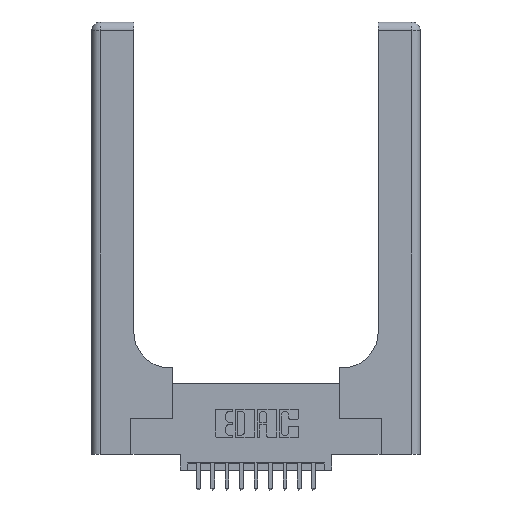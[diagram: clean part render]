
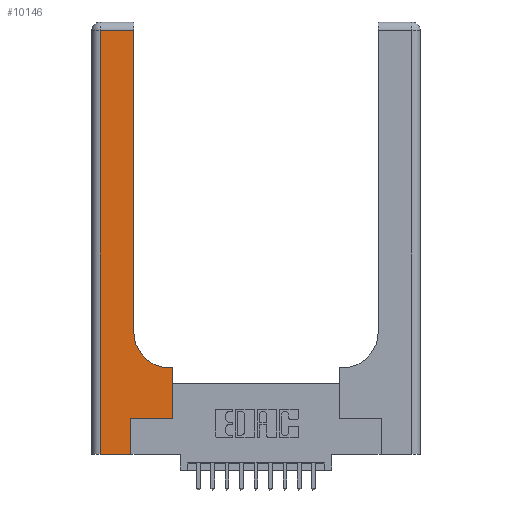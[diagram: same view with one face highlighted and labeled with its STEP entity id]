
A CAD part, top view. The second image highlights one B-rep face of the part: STEP entity #10146.
In plain terms, the highlighted planar face has unit normal (0, 0, 1).
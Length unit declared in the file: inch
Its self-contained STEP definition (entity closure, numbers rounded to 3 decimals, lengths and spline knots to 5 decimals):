
#248 = CARTESIAN_POINT ( 'NONE',  ( 0., 3., 0.37 ) ) ;
#299 = CARTESIAN_POINT ( 'NONE',  ( 0.269, 0., 0.37 ) ) ;
#322 = ORIENTED_EDGE ( 'NONE', *, *, #13835, .T. ) ;
#535 = DIRECTION ( 'NONE',  ( 1., 0., 0. ) ) ;
#1595 = ORIENTED_EDGE ( 'NONE', *, *, #2756, .T. ) ;
#1666 = DIRECTION ( 'NONE',  ( 0., 1., 0. ) ) ;
#1703 = LINE ( 'NONE', #5722, #5166 ) ;
#2018 = ORIENTED_EDGE ( 'NONE', *, *, #13141, .T. ) ;
#2020 = CARTESIAN_POINT ( 'NONE',  ( 0.269, 0.25, 0.37 ) ) ;
#2033 = DIRECTION ( 'NONE',  ( 1., 0., 0. ) ) ;
#2410 = DIRECTION ( 'NONE',  ( 0., 1., 0. ) ) ;
#2480 = CARTESIAN_POINT ( 'NONE',  ( 0.269, 0., 0.37 ) ) ;
#2653 = DIRECTION ( 'NONE',  ( -1., 0., 0. ) ) ;
#2694 = LINE ( 'NONE', #14107, #6536 ) ;
#2756 = EDGE_CURVE ( 'NONE', #9145, #10440, #5710, .T. ) ;
#2919 = DIRECTION ( 'NONE',  ( 0., 0., -1. ) ) ;
#3047 = CARTESIAN_POINT ( 'NONE',  ( 0.5585, 0.6, 0.37 ) ) ;
#3110 = AXIS2_PLACEMENT_3D ( 'NONE', #16132, #8340, #535 ) ;
#3440 = EDGE_CURVE ( 'NONE', #14490, #9145, #13629, .T. ) ;
#3652 = CARTESIAN_POINT ( 'NONE',  ( 0.2915, 3., 0.37 ) ) ;
#4096 = VECTOR ( 'NONE', #12727, 39.37008 ) ;
#4307 = CARTESIAN_POINT ( 'NONE',  ( 0., 0., 0.37 ) ) ;
#4726 = VERTEX_POINT ( 'NONE', #3047 ) ;
#5166 = VECTOR ( 'NONE', #14821, 39.37008 ) ;
#5465 = ORIENTED_EDGE ( 'NONE', *, *, #7130, .T. ) ;
#5710 = LINE ( 'NONE', #2020, #11809 ) ;
#5722 = CARTESIAN_POINT ( 'NONE',  ( 0.2915, 0.6, 0.37 ) ) ;
#5902 = CARTESIAN_POINT ( 'NONE',  ( 0.269, 0.25, 0.37 ) ) ;
#6536 = VECTOR ( 'NONE', #2410, 39.37008 ) ;
#6559 = LINE ( 'NONE', #12998, #13080 ) ;
#6918 = DIRECTION ( 'NONE',  ( 1., 0., 0. ) ) ;
#7130 = EDGE_CURVE ( 'NONE', #4726, #11385, #1703, .T. ) ;
#7394 = CARTESIAN_POINT ( 'NONE',  ( 0.06, 2.94, 0.37 ) ) ;
#7572 = EDGE_LOOP ( 'NONE', ( #322, #14205, #7686, #11154, #8086, #1595, #2018, #5465, #15815 ) ) ;
#7686 = ORIENTED_EDGE ( 'NONE', *, *, #9153, .T. ) ;
#8086 = ORIENTED_EDGE ( 'NONE', *, *, #3440, .T. ) ;
#8340 = DIRECTION ( 'NONE',  ( 0., 0., -1. ) ) ;
#8570 = CARTESIAN_POINT ( 'NONE',  ( 0.5585, 0.25, 0.37 ) ) ;
#8605 = EDGE_CURVE ( 'NONE', #11385, #11068, #15018, .T. ) ;
#9145 = VERTEX_POINT ( 'NONE', #5902 ) ;
#9153 = EDGE_CURVE ( 'NONE', #13086, #14885, #10295, .T. ) ;
#9863 = FACE_OUTER_BOUND ( 'NONE', #7572, .T. ) ;
#10146 = ADVANCED_FACE ( 'NONE', ( #9863 ), #14574, .F. ) ;
#10153 = VECTOR ( 'NONE', #1666, 39.37008 ) ;
#10295 = LINE ( 'NONE', #12380, #12951 ) ;
#10440 = VERTEX_POINT ( 'NONE', #8570 ) ;
#11068 = VERTEX_POINT ( 'NONE', #16280 ) ;
#11154 = ORIENTED_EDGE ( 'NONE', *, *, #15310, .T. ) ;
#11385 = VERTEX_POINT ( 'NONE', #11429 ) ;
#11429 = CARTESIAN_POINT ( 'NONE',  ( 0.5415, 0.6, 0.37 ) ) ;
#11809 = VECTOR ( 'NONE', #2033, 39.37008 ) ;
#12004 = DIRECTION ( 'NONE',  ( -1., 0., 0. ) ) ;
#12380 = CARTESIAN_POINT ( 'NONE',  ( 0.06, 3., 0.37 ) ) ;
#12570 = CARTESIAN_POINT ( 'NONE',  ( 0.06, 0., 0.37 ) ) ;
#12657 = EDGE_CURVE ( 'NONE', #15688, #13086, #6559, .T. ) ;
#12682 = VECTOR ( 'NONE', #6918, 39.37008 ) ;
#12727 = DIRECTION ( 'NONE',  ( 0., 1., 0. ) ) ;
#12951 = VECTOR ( 'NONE', #16278, 39.37008 ) ;
#12998 = CARTESIAN_POINT ( 'NONE',  ( 0., 2.94, 0.37 ) ) ;
#13080 = VECTOR ( 'NONE', #2653, 39.37008 ) ;
#13086 = VERTEX_POINT ( 'NONE', #7394 ) ;
#13141 = EDGE_CURVE ( 'NONE', #10440, #4726, #2694, .T. ) ;
#13228 = CARTESIAN_POINT ( 'NONE',  ( 0.2915, 2.94, 0.37 ) ) ;
#13629 = LINE ( 'NONE', #299, #10153 ) ;
#13835 = EDGE_CURVE ( 'NONE', #11068, #15688, #14045, .T. ) ;
#14045 = LINE ( 'NONE', #3652, #4096 ) ;
#14107 = CARTESIAN_POINT ( 'NONE',  ( 0.5585, 0.25, 0.37 ) ) ;
#14205 = ORIENTED_EDGE ( 'NONE', *, *, #12657, .T. ) ;
#14490 = VERTEX_POINT ( 'NONE', #2480 ) ;
#14574 = PLANE ( 'NONE',  #16583 ) ;
#14821 = DIRECTION ( 'NONE',  ( -1., 0., 0. ) ) ;
#14885 = VERTEX_POINT ( 'NONE', #12570 ) ;
#15018 = CIRCLE ( 'NONE', #3110, 0.25 ) ;
#15310 = EDGE_CURVE ( 'NONE', #14885, #14490, #16506, .T. ) ;
#15688 = VERTEX_POINT ( 'NONE', #13228 ) ;
#15815 = ORIENTED_EDGE ( 'NONE', *, *, #8605, .T. ) ;
#16132 = CARTESIAN_POINT ( 'NONE',  ( 0.5415, 0.85, 0.37 ) ) ;
#16278 = DIRECTION ( 'NONE',  ( 0., -1., 0. ) ) ;
#16280 = CARTESIAN_POINT ( 'NONE',  ( 0.2915, 0.85, 0.37 ) ) ;
#16506 = LINE ( 'NONE', #4307, #12682 ) ;
#16583 = AXIS2_PLACEMENT_3D ( 'NONE', #248, #2919, #12004 ) ;
